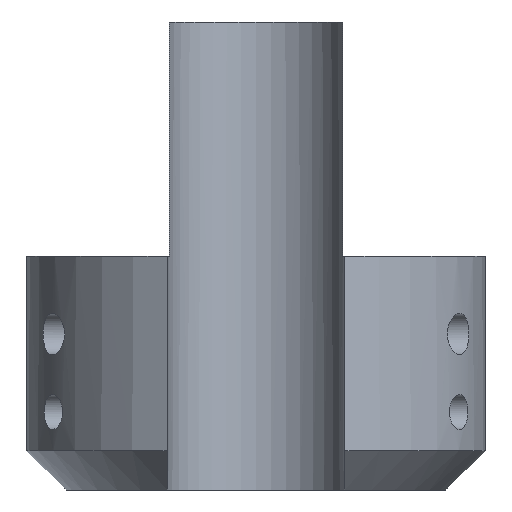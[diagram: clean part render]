
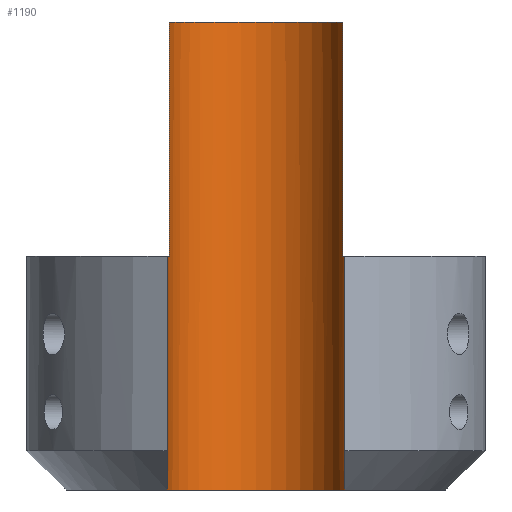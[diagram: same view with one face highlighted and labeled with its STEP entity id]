
A CAD part, left-side view. The second image highlights one B-rep face of the part: STEP entity #1190.
In plain terms, the highlighted cylindrical face has radius 7.239 mm (diameter 14.478 mm), a partial arc.
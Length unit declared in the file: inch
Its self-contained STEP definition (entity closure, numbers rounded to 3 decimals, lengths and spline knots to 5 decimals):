
#9 = EDGE_CURVE ( 'NONE', #1197, #738, #633, .T. ) ;
#20 = DIRECTION ( 'NONE',  ( -1., 0., 0. ) ) ;
#23 = CARTESIAN_POINT ( 'NONE',  ( 0.06278, -0.278, 0.75 ) ) ;
#34 = AXIS2_PLACEMENT_3D ( 'NONE', #1045, #471, #285 ) ;
#55 = CARTESIAN_POINT ( 'NONE',  ( 0., 0., 0.75 ) ) ;
#61 = CARTESIAN_POINT ( 'NONE',  ( 0.06278, -0.278, 1.5 ) ) ;
#62 = ORIENTED_EDGE ( 'NONE', *, *, #727, .F. ) ;
#90 = EDGE_CURVE ( 'NONE', #1018, #245, #154, .T. ) ;
#93 = DIRECTION ( 'NONE',  ( 0., 0., -1. ) ) ;
#154 = CIRCLE ( 'NONE', #34, 0.285 ) ;
#156 = EDGE_CURVE ( 'NONE', #1197, #1018, #989, .T. ) ;
#210 = DIRECTION ( 'NONE',  ( -1., 0., 0. ) ) ;
#212 = AXIS2_PLACEMENT_3D ( 'NONE', #1169, #791, #210 ) ;
#238 = CARTESIAN_POINT ( 'NONE',  ( 0., 0., 0.75 ) ) ;
#245 = VERTEX_POINT ( 'NONE', #399 ) ;
#269 = VECTOR ( 'NONE', #93, 39.37008 ) ;
#285 = DIRECTION ( 'NONE',  ( 1., 0., 0. ) ) ;
#307 = VECTOR ( 'NONE', #387, 39.37008 ) ;
#310 = VERTEX_POINT ( 'NONE', #965 ) ;
#326 = VECTOR ( 'NONE', #1156, 39.37008 ) ;
#351 = EDGE_CURVE ( 'NONE', #1099, #778, #913, .T. ) ;
#354 = DIRECTION ( 'NONE',  ( 0., 0., -1. ) ) ;
#370 = VERTEX_POINT ( 'NONE', #23 ) ;
#385 = ORIENTED_EDGE ( 'NONE', *, *, #1214, .T. ) ;
#387 = DIRECTION ( 'NONE',  ( 0., 0., -1. ) ) ;
#392 = CARTESIAN_POINT ( 'NONE',  ( 0.06278, 0.278, 0.75 ) ) ;
#399 = CARTESIAN_POINT ( 'NONE',  ( 0., -0.285, 0. ) ) ;
#401 = CARTESIAN_POINT ( 'NONE',  ( 0., 0.285, 0.75 ) ) ;
#420 = LINE ( 'NONE', #61, #806 ) ;
#432 = DIRECTION ( 'NONE',  ( 1., 0., 0. ) ) ;
#433 = LINE ( 'NONE', #1239, #269 ) ;
#461 = ORIENTED_EDGE ( 'NONE', *, *, #676, .F. ) ;
#470 = ORIENTED_EDGE ( 'NONE', *, *, #911, .F. ) ;
#471 = DIRECTION ( 'NONE',  ( 0., 0., -1. ) ) ;
#492 = ORIENTED_EDGE ( 'NONE', *, *, #90, .T. ) ;
#494 = CARTESIAN_POINT ( 'NONE',  ( 0.06278, -0.278, 1.5 ) ) ;
#518 = AXIS2_PLACEMENT_3D ( 'NONE', #524, #1175, #20 ) ;
#524 = CARTESIAN_POINT ( 'NONE',  ( 0., 0., 1.5 ) ) ;
#568 = CIRCLE ( 'NONE', #689, 0.285 ) ;
#575 = CARTESIAN_POINT ( 'NONE',  ( 0.06278, 0.278, 1.5 ) ) ;
#613 = DIRECTION ( 'NONE',  ( 1., 0., 0. ) ) ;
#633 = CIRCLE ( 'NONE', #1050, 0.285 ) ;
#663 = CARTESIAN_POINT ( 'NONE',  ( 0., 0.285, 0. ) ) ;
#676 = EDGE_CURVE ( 'NONE', #778, #370, #420, .T. ) ;
#681 = CARTESIAN_POINT ( 'NONE',  ( 0.06278, 0.278, 1.5 ) ) ;
#689 = AXIS2_PLACEMENT_3D ( 'NONE', #55, #354, #432 ) ;
#696 = ORIENTED_EDGE ( 'NONE', *, *, #9, .F. ) ;
#727 = EDGE_CURVE ( 'NONE', #310, #245, #433, .T. ) ;
#738 = VERTEX_POINT ( 'NONE', #392 ) ;
#767 = LINE ( 'NONE', #681, #326 ) ;
#778 = VERTEX_POINT ( 'NONE', #494 ) ;
#791 = DIRECTION ( 'NONE',  ( 0., 0., -1. ) ) ;
#806 = VECTOR ( 'NONE', #1022, 39.37008 ) ;
#858 = EDGE_LOOP ( 'NONE', ( #492, #62, #470, #461, #917, #385, #696, #916 ) ) ;
#884 = CYLINDRICAL_SURFACE ( 'NONE', #212, 0.285 ) ;
#911 = EDGE_CURVE ( 'NONE', #370, #310, #568, .T. ) ;
#913 = CIRCLE ( 'NONE', #518, 0.285 ) ;
#916 = ORIENTED_EDGE ( 'NONE', *, *, #156, .T. ) ;
#917 = ORIENTED_EDGE ( 'NONE', *, *, #351, .F. ) ;
#932 = FACE_OUTER_BOUND ( 'NONE', #858, .T. ) ;
#965 = CARTESIAN_POINT ( 'NONE',  ( 0., -0.285, 0.75 ) ) ;
#989 = LINE ( 'NONE', #1134, #307 ) ;
#1018 = VERTEX_POINT ( 'NONE', #663 ) ;
#1022 = DIRECTION ( 'NONE',  ( 0., 0., -1. ) ) ;
#1045 = CARTESIAN_POINT ( 'NONE',  ( 0., 0., 0. ) ) ;
#1050 = AXIS2_PLACEMENT_3D ( 'NONE', #238, #1191, #613 ) ;
#1099 = VERTEX_POINT ( 'NONE', #575 ) ;
#1134 = CARTESIAN_POINT ( 'NONE',  ( 0., 0.285, 0.75 ) ) ;
#1156 = DIRECTION ( 'NONE',  ( 0., 0., -1. ) ) ;
#1169 = CARTESIAN_POINT ( 'NONE',  ( 0., 0., 0.75 ) ) ;
#1175 = DIRECTION ( 'NONE',  ( 0., 0., -1. ) ) ;
#1190 = ADVANCED_FACE ( 'NONE', ( #932 ), #884, .F. ) ;
#1191 = DIRECTION ( 'NONE',  ( 0., 0., -1. ) ) ;
#1197 = VERTEX_POINT ( 'NONE', #401 ) ;
#1214 = EDGE_CURVE ( 'NONE', #1099, #738, #767, .T. ) ;
#1239 = CARTESIAN_POINT ( 'NONE',  ( 0., -0.285, 0.75 ) ) ;
